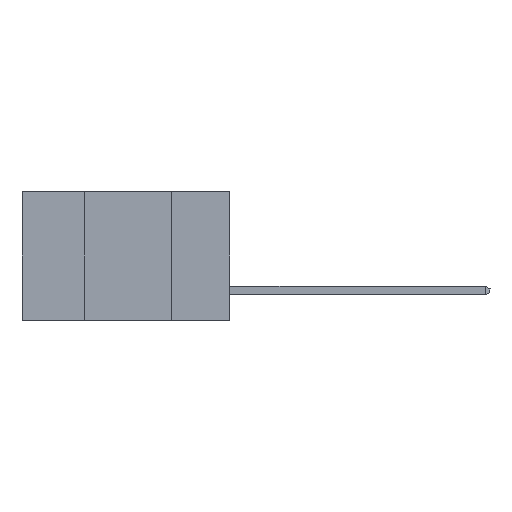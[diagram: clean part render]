
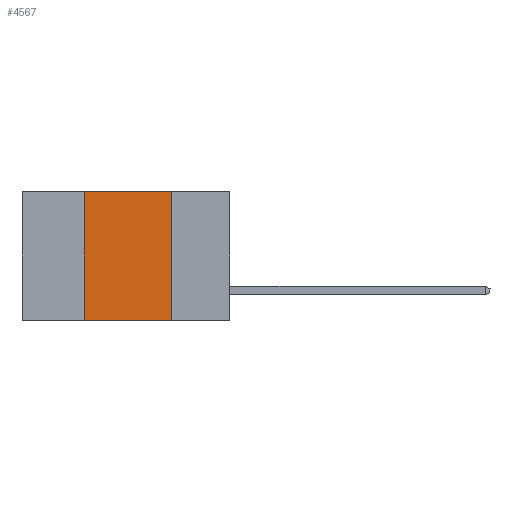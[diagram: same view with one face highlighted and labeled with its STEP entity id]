
A CAD part, left-side view. The second image highlights one B-rep face of the part: STEP entity #4567.
In plain terms, the highlighted planar face has unit normal (-1, 0, 0).
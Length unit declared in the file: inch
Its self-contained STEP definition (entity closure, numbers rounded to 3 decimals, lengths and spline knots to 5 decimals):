
#39 = CARTESIAN_POINT ( 'NONE',  ( 0., 0.17, -0.37 ) ) ;
#1806 = EDGE_CURVE ( 'NONE', #3528, #9512, #17762, .T. ) ;
#2689 = VECTOR ( 'NONE', #5025, 39.37008 ) ;
#2849 = LINE ( 'NONE', #11861, #3458 ) ;
#3341 = DIRECTION ( 'NONE',  ( 1., 0., 0. ) ) ;
#3458 = VECTOR ( 'NONE', #17847, 39.37008 ) ;
#3528 = VERTEX_POINT ( 'NONE', #7078 ) ;
#4330 = CARTESIAN_POINT ( 'NONE',  ( 0., 0.6, -0.37 ) ) ;
#4567 = ADVANCED_FACE ( 'NONE', ( #16665 ), #16767, .F. ) ;
#4993 = CARTESIAN_POINT ( 'NONE',  ( 0., 0.42, -0.37 ) ) ;
#5025 = DIRECTION ( 'NONE',  ( 0., -1., 0. ) ) ;
#6142 = ORIENTED_EDGE ( 'NONE', *, *, #11531, .F. ) ;
#6292 = EDGE_CURVE ( 'NONE', #13672, #9512, #2849, .T. ) ;
#6298 = AXIS2_PLACEMENT_3D ( 'NONE', #11975, #3341, #17962 ) ;
#7078 = CARTESIAN_POINT ( 'NONE',  ( 0., 0.42, -0.37 ) ) ;
#7120 = VERTEX_POINT ( 'NONE', #15230 ) ;
#7394 = VECTOR ( 'NONE', #11071, 39.37008 ) ;
#8842 = DIRECTION ( 'NONE',  ( 0., -1., 0. ) ) ;
#9512 = VERTEX_POINT ( 'NONE', #39 ) ;
#9881 = LINE ( 'NONE', #4993, #7394 ) ;
#10934 = VECTOR ( 'NONE', #8842, 39.37008 ) ;
#11071 = DIRECTION ( 'NONE',  ( 0., 0., 1. ) ) ;
#11531 = EDGE_CURVE ( 'NONE', #7120, #13672, #13915, .T. ) ;
#11566 = EDGE_LOOP ( 'NONE', ( #11873, #6142, #12410, #17311 ) ) ;
#11861 = CARTESIAN_POINT ( 'NONE',  ( 0., 0.17, -0.37 ) ) ;
#11873 = ORIENTED_EDGE ( 'NONE', *, *, #6292, .F. ) ;
#11975 = CARTESIAN_POINT ( 'NONE',  ( 0., 0.6, 0. ) ) ;
#12410 = ORIENTED_EDGE ( 'NONE', *, *, #13818, .F. ) ;
#12541 = CARTESIAN_POINT ( 'NONE',  ( 0., 0.6, 0. ) ) ;
#13510 = CARTESIAN_POINT ( 'NONE',  ( 0., 0.17, 0. ) ) ;
#13672 = VERTEX_POINT ( 'NONE', #13510 ) ;
#13818 = EDGE_CURVE ( 'NONE', #3528, #7120, #9881, .T. ) ;
#13915 = LINE ( 'NONE', #12541, #2689 ) ;
#15230 = CARTESIAN_POINT ( 'NONE',  ( 0., 0.42, 0. ) ) ;
#16665 = FACE_OUTER_BOUND ( 'NONE', #11566, .T. ) ;
#16767 = PLANE ( 'NONE',  #6298 ) ;
#17311 = ORIENTED_EDGE ( 'NONE', *, *, #1806, .T. ) ;
#17762 = LINE ( 'NONE', #4330, #10934 ) ;
#17847 = DIRECTION ( 'NONE',  ( 0., 0., -1. ) ) ;
#17962 = DIRECTION ( 'NONE',  ( 0., 0., -1. ) ) ;
